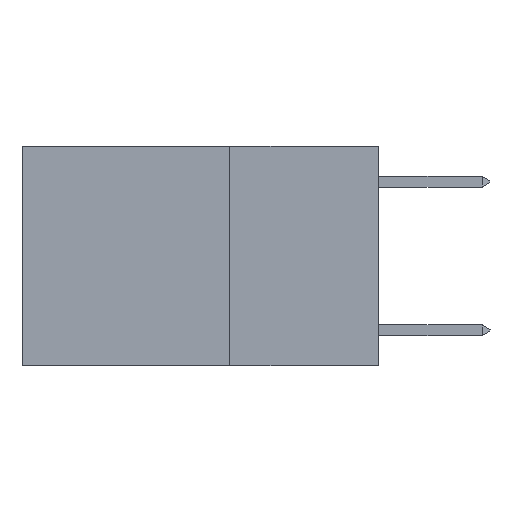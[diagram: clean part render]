
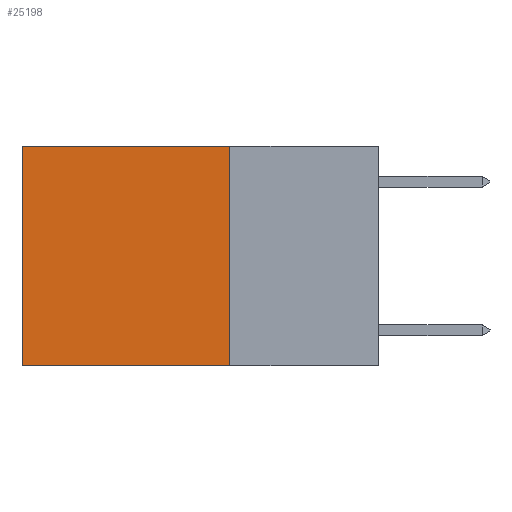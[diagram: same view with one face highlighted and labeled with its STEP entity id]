
A CAD part, left-side view. The second image highlights one B-rep face of the part: STEP entity #25198.
In plain terms, the highlighted planar face has unit normal (-1, 0, 0).
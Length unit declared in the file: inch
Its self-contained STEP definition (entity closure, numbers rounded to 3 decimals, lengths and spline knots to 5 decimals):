
#13 = DIRECTION ( 'NONE',  ( 0., 1., 0. ) ) ;
#1417 = CARTESIAN_POINT ( 'NONE',  ( 0.2625, 0.25, 0. ) ) ;
#5167 = CARTESIAN_POINT ( 'NONE',  ( 0.2625, 0.25, 0. ) ) ;
#5205 = DIRECTION ( 'NONE',  ( 0., 0., -1. ) ) ;
#7151 = CARTESIAN_POINT ( 'NONE',  ( 0.2625, 0.6, 0. ) ) ;
#8803 = PLANE ( 'NONE',  #26861 ) ;
#9201 = VERTEX_POINT ( 'NONE', #22380 ) ;
#11331 = DIRECTION ( 'NONE',  ( 0., 0., -1. ) ) ;
#11404 = EDGE_CURVE ( 'NONE', #15612, #21867, #18157, .T. ) ;
#11726 = VECTOR ( 'NONE', #5205, 39.37008 ) ;
#12456 = LINE ( 'NONE', #29545, #11726 ) ;
#13023 = VECTOR ( 'NONE', #24973, 39.37008 ) ;
#13179 = ORIENTED_EDGE ( 'NONE', *, *, #24882, .F. ) ;
#13679 = ORIENTED_EDGE ( 'NONE', *, *, #27847, .F. ) ;
#14541 = VECTOR ( 'NONE', #13, 39.37008 ) ;
#15612 = VERTEX_POINT ( 'NONE', #5167 ) ;
#16262 = VERTEX_POINT ( 'NONE', #27185 ) ;
#16986 = FACE_OUTER_BOUND ( 'NONE', #21849, .T. ) ;
#17144 = CARTESIAN_POINT ( 'NONE',  ( 0.2625, 0.25, -0.37 ) ) ;
#17620 = CARTESIAN_POINT ( 'NONE',  ( 0.2625, 0.6, 0. ) ) ;
#18011 = VECTOR ( 'NONE', #23991, 39.37008 ) ;
#18157 = LINE ( 'NONE', #23881, #18011 ) ;
#20259 = LINE ( 'NONE', #17620, #13023 ) ;
#21394 = EDGE_CURVE ( 'NONE', #21867, #9201, #20259, .T. ) ;
#21605 = ORIENTED_EDGE ( 'NONE', *, *, #11404, .T. ) ;
#21794 = LINE ( 'NONE', #17144, #14541 ) ;
#21849 = EDGE_LOOP ( 'NONE', ( #30608, #13679, #13179, #21605 ) ) ;
#21867 = VERTEX_POINT ( 'NONE', #7151 ) ;
#22380 = CARTESIAN_POINT ( 'NONE',  ( 0.2625, 0.6, -0.37 ) ) ;
#23881 = CARTESIAN_POINT ( 'NONE',  ( 0.2625, 0.25, 0. ) ) ;
#23991 = DIRECTION ( 'NONE',  ( 0., 1., 0. ) ) ;
#24882 = EDGE_CURVE ( 'NONE', #15612, #16262, #12456, .T. ) ;
#24973 = DIRECTION ( 'NONE',  ( 0., 0., -1. ) ) ;
#25198 = ADVANCED_FACE ( 'NONE', ( #16986 ), #8803, .F. ) ;
#25856 = DIRECTION ( 'NONE',  ( 1., 0., 0. ) ) ;
#26861 = AXIS2_PLACEMENT_3D ( 'NONE', #1417, #25856, #11331 ) ;
#27185 = CARTESIAN_POINT ( 'NONE',  ( 0.2625, 0.25, -0.37 ) ) ;
#27847 = EDGE_CURVE ( 'NONE', #16262, #9201, #21794, .T. ) ;
#29545 = CARTESIAN_POINT ( 'NONE',  ( 0.2625, 0.25, 0. ) ) ;
#30608 = ORIENTED_EDGE ( 'NONE', *, *, #21394, .T. ) ;
